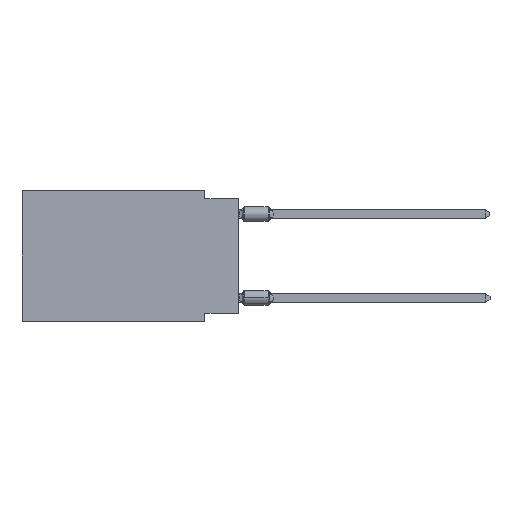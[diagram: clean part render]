
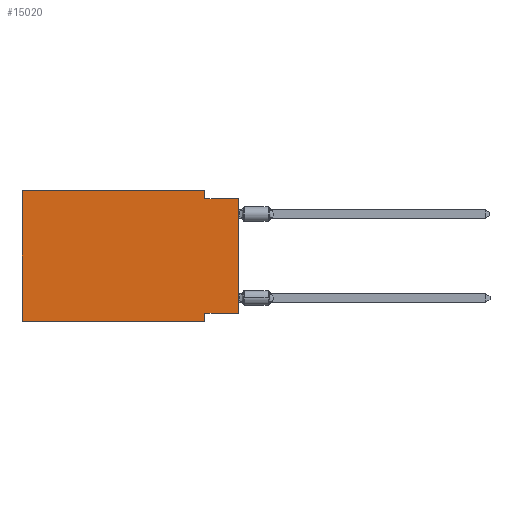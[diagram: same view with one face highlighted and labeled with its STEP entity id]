
A CAD part, left-side view. The second image highlights one B-rep face of the part: STEP entity #15020.
In plain terms, the highlighted planar face has unit normal (-1, 0, 0).
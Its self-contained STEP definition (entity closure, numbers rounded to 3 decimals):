
#29 = VERTEX_POINT ( 'NONE', #16460 ) ;
#378 = AXIS2_PLACEMENT_3D ( 'NONE', #16880, #11883, #12190 ) ;
#433 = EDGE_CURVE ( 'NONE', #3956, #29, #5251, .T. ) ;
#647 = PLANE ( 'NONE',  #378 ) ;
#745 = VECTOR ( 'NONE', #1694, 1000. ) ;
#1314 = ORIENTED_EDGE ( 'NONE', *, *, #7243, .F. ) ;
#1559 = LINE ( 'NONE', #3287, #9502 ) ;
#1694 = DIRECTION ( 'NONE',  ( 0., 0., 1. ) ) ;
#2299 = VECTOR ( 'NONE', #2400, 1000. ) ;
#2367 = ORIENTED_EDGE ( 'NONE', *, *, #18574, .F. ) ;
#2400 = DIRECTION ( 'NONE',  ( 0., 0., 1. ) ) ;
#2890 = EDGE_CURVE ( 'NONE', #9243, #16605, #7639, .T. ) ;
#3287 = CARTESIAN_POINT ( 'NONE',  ( 0., 2.54, 0. ) ) ;
#3321 = DIRECTION ( 'NONE',  ( 0., -1., 0. ) ) ;
#3703 = LINE ( 'NONE', #15471, #2299 ) ;
#3886 = FACE_OUTER_BOUND ( 'NONE', #5443, .T. ) ;
#3956 = VERTEX_POINT ( 'NONE', #12702 ) ;
#4047 = ORIENTED_EDGE ( 'NONE', *, *, #9743, .F. ) ;
#4246 = VECTOR ( 'NONE', #15660, 1000. ) ;
#5071 = CARTESIAN_POINT ( 'NONE',  ( 0., 0., -9.271 ) ) ;
#5251 = LINE ( 'NONE', #13132, #7280 ) ;
#5443 = EDGE_LOOP ( 'NONE', ( #8511, #6002, #2367, #12372, #4047, #9709, #1314, #13951 ) ) ;
#5533 = DIRECTION ( 'NONE',  ( 0., -1., 0. ) ) ;
#6002 = ORIENTED_EDGE ( 'NONE', *, *, #2890, .F. ) ;
#6366 = CARTESIAN_POINT ( 'NONE',  ( 0., 0., -9.271 ) ) ;
#6382 = CARTESIAN_POINT ( 'NONE',  ( 0., 16.383, -9.906 ) ) ;
#6735 = VECTOR ( 'NONE', #20962, 1000. ) ;
#7243 = EDGE_CURVE ( 'NONE', #19391, #8285, #19131, .T. ) ;
#7280 = VECTOR ( 'NONE', #3321, 1000. ) ;
#7639 = LINE ( 'NONE', #14026, #6735 ) ;
#8285 = VERTEX_POINT ( 'NONE', #19483 ) ;
#8298 = DIRECTION ( 'NONE',  ( 0., 1., 0. ) ) ;
#8511 = ORIENTED_EDGE ( 'NONE', *, *, #15754, .T. ) ;
#8766 = VERTEX_POINT ( 'NONE', #6366 ) ;
#9243 = VERTEX_POINT ( 'NONE', #15173 ) ;
#9502 = VECTOR ( 'NONE', #15159, 1000. ) ;
#9709 = ORIENTED_EDGE ( 'NONE', *, *, #19742, .T. ) ;
#9743 = EDGE_CURVE ( 'NONE', #14810, #3956, #3703, .T. ) ;
#11883 = DIRECTION ( 'NONE',  ( 1., 0., 0. ) ) ;
#12190 = DIRECTION ( 'NONE',  ( 0., 0., -1. ) ) ;
#12372 = ORIENTED_EDGE ( 'NONE', *, *, #433, .F. ) ;
#12702 = CARTESIAN_POINT ( 'NONE',  ( 0., 16.383, 0. ) ) ;
#13132 = CARTESIAN_POINT ( 'NONE',  ( 0., 16.383, 0. ) ) ;
#13229 = LINE ( 'NONE', #16391, #745 ) ;
#13951 = ORIENTED_EDGE ( 'NONE', *, *, #16580, .F. ) ;
#14026 = CARTESIAN_POINT ( 'NONE',  ( 0., 0., -0.635 ) ) ;
#14680 = VECTOR ( 'NONE', #5533, 1000. ) ;
#14810 = VERTEX_POINT ( 'NONE', #6382 ) ;
#15020 = ADVANCED_FACE ( 'NONE', ( #3886 ), #647, .F. ) ;
#15159 = DIRECTION ( 'NONE',  ( 0., 0., -1. ) ) ;
#15173 = CARTESIAN_POINT ( 'NONE',  ( 0., 2.54, -0.635 ) ) ;
#15260 = CARTESIAN_POINT ( 'NONE',  ( 0., 16.383, -9.906 ) ) ;
#15471 = CARTESIAN_POINT ( 'NONE',  ( 0., 16.383, 0. ) ) ;
#15660 = DIRECTION ( 'NONE',  ( 0., 0., -1. ) ) ;
#15754 = EDGE_CURVE ( 'NONE', #8766, #16605, #13229, .T. ) ;
#16391 = CARTESIAN_POINT ( 'NONE',  ( 0., 0., 0. ) ) ;
#16460 = CARTESIAN_POINT ( 'NONE',  ( 0., 2.54, 0. ) ) ;
#16580 = EDGE_CURVE ( 'NONE', #8766, #19391, #16747, .T. ) ;
#16605 = VERTEX_POINT ( 'NONE', #16637 ) ;
#16637 = CARTESIAN_POINT ( 'NONE',  ( 0., 0., -0.635 ) ) ;
#16747 = LINE ( 'NONE', #5071, #18387 ) ;
#16880 = CARTESIAN_POINT ( 'NONE',  ( 0., 16.383, 0. ) ) ;
#17321 = LINE ( 'NONE', #15260, #14680 ) ;
#18387 = VECTOR ( 'NONE', #8298, 1000. ) ;
#18574 = EDGE_CURVE ( 'NONE', #29, #9243, #1559, .T. ) ;
#19131 = LINE ( 'NONE', #20433, #4246 ) ;
#19391 = VERTEX_POINT ( 'NONE', #20807 ) ;
#19483 = CARTESIAN_POINT ( 'NONE',  ( 0., 2.54, -9.906 ) ) ;
#19742 = EDGE_CURVE ( 'NONE', #14810, #8285, #17321, .T. ) ;
#20433 = CARTESIAN_POINT ( 'NONE',  ( 0., 2.54, -9.906 ) ) ;
#20807 = CARTESIAN_POINT ( 'NONE',  ( 0., 2.54, -9.271 ) ) ;
#20962 = DIRECTION ( 'NONE',  ( 0., -1., 0. ) ) ;
